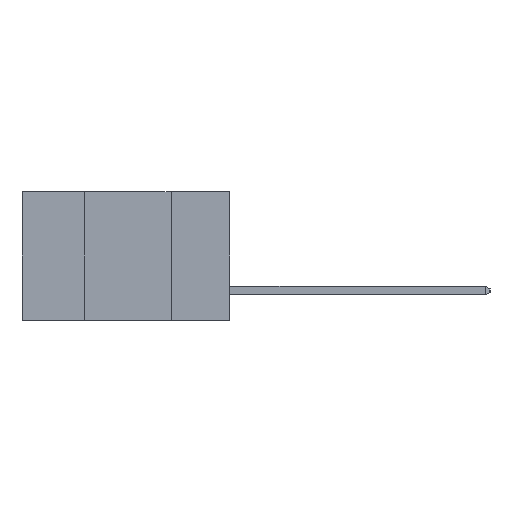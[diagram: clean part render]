
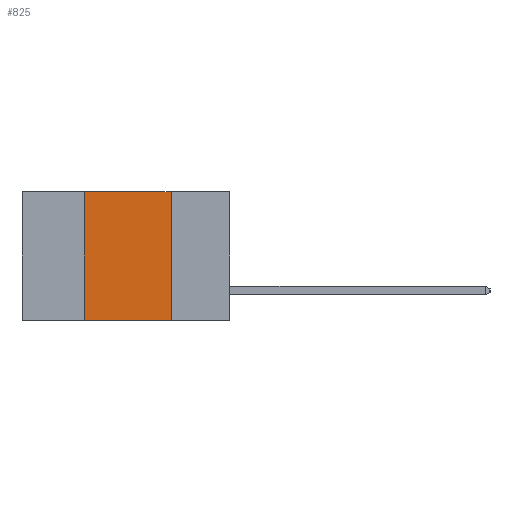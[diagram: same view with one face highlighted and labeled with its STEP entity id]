
A CAD part, left-side view. The second image highlights one B-rep face of the part: STEP entity #825.
In plain terms, the highlighted planar face has unit normal (-1, 0, 0).
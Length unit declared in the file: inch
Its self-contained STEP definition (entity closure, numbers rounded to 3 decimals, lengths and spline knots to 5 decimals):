
#93 = LINE ( 'NONE', #9549, #392 ) ;
#392 = VECTOR ( 'NONE', #10333, 39.37008 ) ;
#720 = LINE ( 'NONE', #2825, #5204 ) ;
#825 = ADVANCED_FACE ( 'NONE', ( #5727 ), #5064, .F. ) ;
#880 = EDGE_CURVE ( 'NONE', #10769, #8797, #720, .T. ) ;
#1018 = VECTOR ( 'NONE', #9017, 39.37008 ) ;
#1897 = EDGE_LOOP ( 'NONE', ( #8242, #10355, #4137, #6654 ) ) ;
#1924 = VERTEX_POINT ( 'NONE', #2100 ) ;
#2100 = CARTESIAN_POINT ( 'NONE',  ( 0., 0.42, 0. ) ) ;
#2444 = EDGE_CURVE ( 'NONE', #1924, #5157, #8172, .T. ) ;
#2825 = CARTESIAN_POINT ( 'NONE',  ( 0., 0.6, -0.37 ) ) ;
#4137 = ORIENTED_EDGE ( 'NONE', *, *, #5463, .F. ) ;
#4607 = AXIS2_PLACEMENT_3D ( 'NONE', #7363, #7638, #4808 ) ;
#4754 = DIRECTION ( 'NONE',  ( 0., -1., 0. ) ) ;
#4808 = DIRECTION ( 'NONE',  ( 0., 0., -1. ) ) ;
#5064 = PLANE ( 'NONE',  #4607 ) ;
#5157 = VERTEX_POINT ( 'NONE', #10746 ) ;
#5204 = VECTOR ( 'NONE', #4754, 39.37008 ) ;
#5463 = EDGE_CURVE ( 'NONE', #10769, #1924, #93, .T. ) ;
#5727 = FACE_OUTER_BOUND ( 'NONE', #1897, .T. ) ;
#5731 = LINE ( 'NONE', #8191, #1018 ) ;
#6626 = CARTESIAN_POINT ( 'NONE',  ( 0., 0.17, -0.37 ) ) ;
#6654 = ORIENTED_EDGE ( 'NONE', *, *, #880, .T. ) ;
#7363 = CARTESIAN_POINT ( 'NONE',  ( 0., 0.6, 0. ) ) ;
#7638 = DIRECTION ( 'NONE',  ( 1., 0., 0. ) ) ;
#8172 = LINE ( 'NONE', #9466, #9794 ) ;
#8191 = CARTESIAN_POINT ( 'NONE',  ( 0., 0.17, 0. ) ) ;
#8242 = ORIENTED_EDGE ( 'NONE', *, *, #10774, .F. ) ;
#8397 = CARTESIAN_POINT ( 'NONE',  ( 0., 0.42, -0.37 ) ) ;
#8797 = VERTEX_POINT ( 'NONE', #6626 ) ;
#9017 = DIRECTION ( 'NONE',  ( 0., 0., -1. ) ) ;
#9466 = CARTESIAN_POINT ( 'NONE',  ( 0., 0.6, 0. ) ) ;
#9549 = CARTESIAN_POINT ( 'NONE',  ( 0., 0.42, 0. ) ) ;
#9598 = DIRECTION ( 'NONE',  ( 0., -1., 0. ) ) ;
#9794 = VECTOR ( 'NONE', #9598, 39.37008 ) ;
#10333 = DIRECTION ( 'NONE',  ( 0., 0., 1. ) ) ;
#10355 = ORIENTED_EDGE ( 'NONE', *, *, #2444, .F. ) ;
#10746 = CARTESIAN_POINT ( 'NONE',  ( 0., 0.17, 0. ) ) ;
#10769 = VERTEX_POINT ( 'NONE', #8397 ) ;
#10774 = EDGE_CURVE ( 'NONE', #5157, #8797, #5731, .T. ) ;
